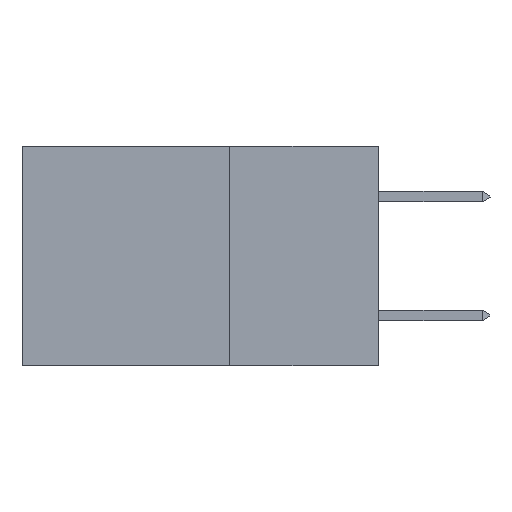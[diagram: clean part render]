
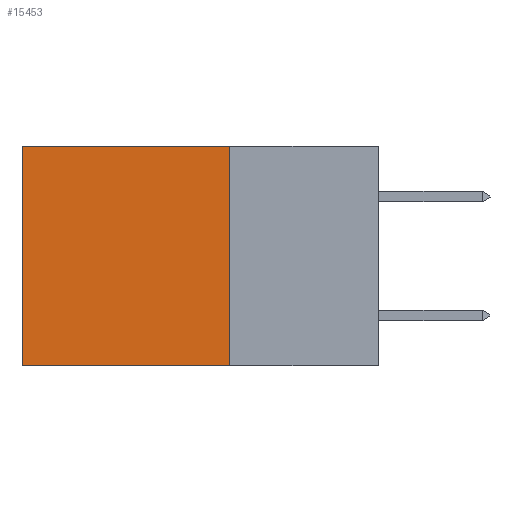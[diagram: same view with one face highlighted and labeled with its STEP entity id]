
A CAD part, left-side view. The second image highlights one B-rep face of the part: STEP entity #15453.
In plain terms, the highlighted planar face has unit normal (-1, 0, 0).
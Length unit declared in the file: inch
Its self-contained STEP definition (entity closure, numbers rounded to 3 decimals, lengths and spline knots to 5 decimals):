
#1085 = VECTOR ( 'NONE', #13498, 39.37008 ) ;
#4100 = CARTESIAN_POINT ( 'NONE',  ( 0.298, 0.25, -0.37 ) ) ;
#5787 = PLANE ( 'NONE',  #10498 ) ;
#6241 = EDGE_LOOP ( 'NONE', ( #16039, #26795, #26696, #17477 ) ) ;
#7727 = DIRECTION ( 'NONE',  ( 0., 0., -1. ) ) ;
#7736 = CARTESIAN_POINT ( 'NONE',  ( 0.298, 0.6, -0.37 ) ) ;
#8614 = LINE ( 'NONE', #26058, #1085 ) ;
#8619 = VERTEX_POINT ( 'NONE', #26986 ) ;
#9593 = EDGE_CURVE ( 'NONE', #8619, #17758, #8614, .T. ) ;
#10282 = CARTESIAN_POINT ( 'NONE',  ( 0.298, 0.6, 0. ) ) ;
#10498 = AXIS2_PLACEMENT_3D ( 'NONE', #20813, #31051, #15913 ) ;
#10504 = VECTOR ( 'NONE', #20385, 39.37008 ) ;
#11039 = VECTOR ( 'NONE', #7727, 39.37008 ) ;
#11508 = EDGE_CURVE ( 'NONE', #8619, #27979, #29876, .T. ) ;
#11592 = DIRECTION ( 'NONE',  ( 0., 1., 0. ) ) ;
#12122 = CARTESIAN_POINT ( 'NONE',  ( 0.298, 0.25, -0.37 ) ) ;
#13446 = VERTEX_POINT ( 'NONE', #7736 ) ;
#13498 = DIRECTION ( 'NONE',  ( 0., 0., -1. ) ) ;
#15066 = CARTESIAN_POINT ( 'NONE',  ( 0.298, 0.6, 0. ) ) ;
#15453 = ADVANCED_FACE ( 'NONE', ( #30168 ), #5787, .F. ) ;
#15631 = EDGE_CURVE ( 'NONE', #17758, #13446, #30542, .T. ) ;
#15913 = DIRECTION ( 'NONE',  ( 0., 0., -1. ) ) ;
#16039 = ORIENTED_EDGE ( 'NONE', *, *, #26729, .T. ) ;
#17477 = ORIENTED_EDGE ( 'NONE', *, *, #11508, .T. ) ;
#17758 = VERTEX_POINT ( 'NONE', #12122 ) ;
#17915 = CARTESIAN_POINT ( 'NONE',  ( 0.298, 0.25, 0. ) ) ;
#19459 = VECTOR ( 'NONE', #11592, 39.37008 ) ;
#20385 = DIRECTION ( 'NONE',  ( 0., 1., 0. ) ) ;
#20813 = CARTESIAN_POINT ( 'NONE',  ( 0.298, 0.25, 0. ) ) ;
#23646 = LINE ( 'NONE', #10282, #11039 ) ;
#26058 = CARTESIAN_POINT ( 'NONE',  ( 0.298, 0.25, 0. ) ) ;
#26696 = ORIENTED_EDGE ( 'NONE', *, *, #9593, .F. ) ;
#26729 = EDGE_CURVE ( 'NONE', #27979, #13446, #23646, .T. ) ;
#26795 = ORIENTED_EDGE ( 'NONE', *, *, #15631, .F. ) ;
#26986 = CARTESIAN_POINT ( 'NONE',  ( 0.298, 0.25, 0. ) ) ;
#27979 = VERTEX_POINT ( 'NONE', #15066 ) ;
#29876 = LINE ( 'NONE', #17915, #10504 ) ;
#30168 = FACE_OUTER_BOUND ( 'NONE', #6241, .T. ) ;
#30542 = LINE ( 'NONE', #4100, #19459 ) ;
#31051 = DIRECTION ( 'NONE',  ( 1., 0., 0. ) ) ;
